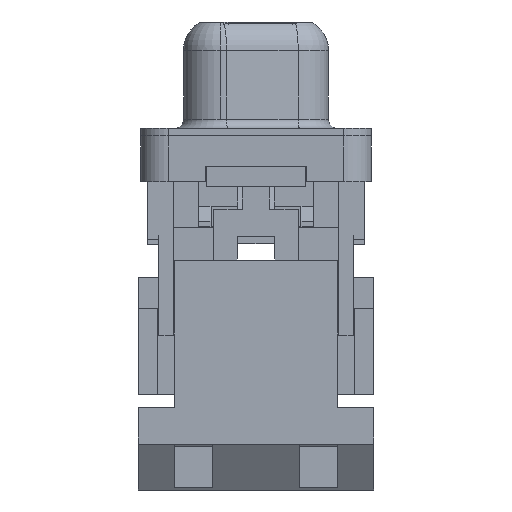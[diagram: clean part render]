
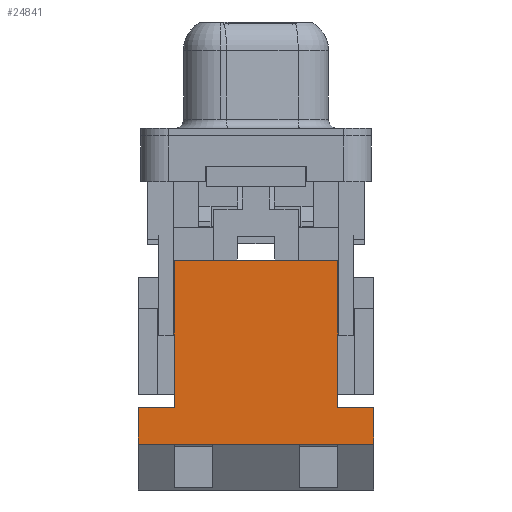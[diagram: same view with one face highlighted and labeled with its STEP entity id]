
A CAD part, left-side view. The second image highlights one B-rep face of the part: STEP entity #24841.
In plain terms, the highlighted planar face has unit normal (-1, 0, 0).
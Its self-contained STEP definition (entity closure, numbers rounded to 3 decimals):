
#735 = CARTESIAN_POINT ( 'NONE',  ( 3.245, 4.45, -6.8 ) ) ;
#1238 = ORIENTED_EDGE ( 'NONE', *, *, #47263, .F. ) ;
#1325 = VERTEX_POINT ( 'NONE', #54065 ) ;
#2243 = VERTEX_POINT ( 'NONE', #48512 ) ;
#4899 = CARTESIAN_POINT ( 'NONE',  ( 3.245, 6.425, -14.8 ) ) ;
#5400 = CARTESIAN_POINT ( 'NONE',  ( 3.245, 6.425, -14.8 ) ) ;
#5487 = EDGE_LOOP ( 'NONE', ( #29639, #77292, #51104, #51401, #29352, #79385, #55973, #1238 ) ) ;
#7276 = CARTESIAN_POINT ( 'NONE',  ( 3.245, -6.425, -16.8 ) ) ;
#7674 = LINE ( 'NONE', #7276, #24705 ) ;
#9521 = LINE ( 'NONE', #22847, #26549 ) ;
#9807 = LINE ( 'NONE', #4899, #60353 ) ;
#10395 = PLANE ( 'NONE',  #64592 ) ;
#18503 = CARTESIAN_POINT ( 'NONE',  ( 3.245, -6.425, -16.8 ) ) ;
#18808 = EDGE_CURVE ( 'NONE', #73652, #64156, #38891, .T. ) ;
#21060 = CARTESIAN_POINT ( 'NONE',  ( 3.245, -6.425, -15.3 ) ) ;
#21924 = EDGE_CURVE ( 'NONE', #69473, #1325, #78391, .T. ) ;
#22847 = CARTESIAN_POINT ( 'NONE',  ( 3.245, 6.425, -15.3 ) ) ;
#22885 = CARTESIAN_POINT ( 'NONE',  ( 3.245, -4.45, -6.8 ) ) ;
#24607 = DIRECTION ( 'NONE',  ( 0., 0., -1. ) ) ;
#24705 = VECTOR ( 'NONE', #74513, 1000. ) ;
#24841 = ADVANCED_FACE ( 'NONE', ( #79210 ), #10395, .F. ) ;
#26549 = VECTOR ( 'NONE', #71857, 1000. ) ;
#27327 = VECTOR ( 'NONE', #67121, 1000. ) ;
#29352 = ORIENTED_EDGE ( 'NONE', *, *, #21924, .F. ) ;
#29639 = ORIENTED_EDGE ( 'NONE', *, *, #79049, .T. ) ;
#31870 = EDGE_CURVE ( 'NONE', #1325, #73652, #49596, .T. ) ;
#36280 = CARTESIAN_POINT ( 'NONE',  ( 3.245, -6.425, -15.3 ) ) ;
#38292 = VECTOR ( 'NONE', #24607, 1000. ) ;
#38891 = LINE ( 'NONE', #21060, #59990 ) ;
#40833 = CARTESIAN_POINT ( 'NONE',  ( 3.245, 4.45, -6.8 ) ) ;
#42766 = VECTOR ( 'NONE', #65762, 1000. ) ;
#43790 = CARTESIAN_POINT ( 'NONE',  ( 3.245, 6.425, -16.8 ) ) ;
#45373 = DIRECTION ( 'NONE',  ( 0., 0., -1. ) ) ;
#47263 = EDGE_CURVE ( 'NONE', #62429, #2243, #9807, .T. ) ;
#47607 = DIRECTION ( 'NONE',  ( 0., 0., -1. ) ) ;
#48250 = DIRECTION ( 'NONE',  ( 0., -1., 0. ) ) ;
#48499 = LINE ( 'NONE', #40833, #27327 ) ;
#48512 = CARTESIAN_POINT ( 'NONE',  ( 3.245, 4.45, -14.8 ) ) ;
#48772 = VERTEX_POINT ( 'NONE', #43790 ) ;
#49322 = LINE ( 'NONE', #735, #38292 ) ;
#49596 = LINE ( 'NONE', #74291, #42766 ) ;
#51027 = CARTESIAN_POINT ( 'NONE',  ( 3.245, -6.425, -14.8 ) ) ;
#51104 = ORIENTED_EDGE ( 'NONE', *, *, #18808, .F. ) ;
#51401 = ORIENTED_EDGE ( 'NONE', *, *, #31870, .F. ) ;
#51471 = VECTOR ( 'NONE', #47607, 1000. ) ;
#52005 = VERTEX_POINT ( 'NONE', #61004 ) ;
#52755 = EDGE_CURVE ( 'NONE', #64156, #48772, #7674, .T. ) ;
#54065 = CARTESIAN_POINT ( 'NONE',  ( 3.245, -4.45, -14.8 ) ) ;
#55973 = ORIENTED_EDGE ( 'NONE', *, *, #63417, .T. ) ;
#59776 = DIRECTION ( 'NONE',  ( 0., 0., -1. ) ) ;
#59990 = VECTOR ( 'NONE', #45373, 1000. ) ;
#60353 = VECTOR ( 'NONE', #48250, 1000. ) ;
#61004 = CARTESIAN_POINT ( 'NONE',  ( 3.245, 4.45, -6.8 ) ) ;
#62429 = VERTEX_POINT ( 'NONE', #5400 ) ;
#63417 = EDGE_CURVE ( 'NONE', #52005, #2243, #49322, .T. ) ;
#64156 = VERTEX_POINT ( 'NONE', #18503 ) ;
#64592 = AXIS2_PLACEMENT_3D ( 'NONE', #36280, #72327, #59776 ) ;
#65762 = DIRECTION ( 'NONE',  ( 0., -1., 0. ) ) ;
#67121 = DIRECTION ( 'NONE',  ( 0., -1., 0. ) ) ;
#67784 = EDGE_CURVE ( 'NONE', #52005, #69473, #48499, .T. ) ;
#69473 = VERTEX_POINT ( 'NONE', #71912 ) ;
#71857 = DIRECTION ( 'NONE',  ( 0., 0., -1. ) ) ;
#71912 = CARTESIAN_POINT ( 'NONE',  ( 3.245, -4.45, -6.8 ) ) ;
#72327 = DIRECTION ( 'NONE',  ( 1., 0., 0. ) ) ;
#73652 = VERTEX_POINT ( 'NONE', #51027 ) ;
#74291 = CARTESIAN_POINT ( 'NONE',  ( 3.245, 6.425, -14.8 ) ) ;
#74513 = DIRECTION ( 'NONE',  ( 0., 1., 0. ) ) ;
#77292 = ORIENTED_EDGE ( 'NONE', *, *, #52755, .F. ) ;
#78391 = LINE ( 'NONE', #22885, #51471 ) ;
#79049 = EDGE_CURVE ( 'NONE', #62429, #48772, #9521, .T. ) ;
#79210 = FACE_OUTER_BOUND ( 'NONE', #5487, .T. ) ;
#79385 = ORIENTED_EDGE ( 'NONE', *, *, #67784, .F. ) ;
